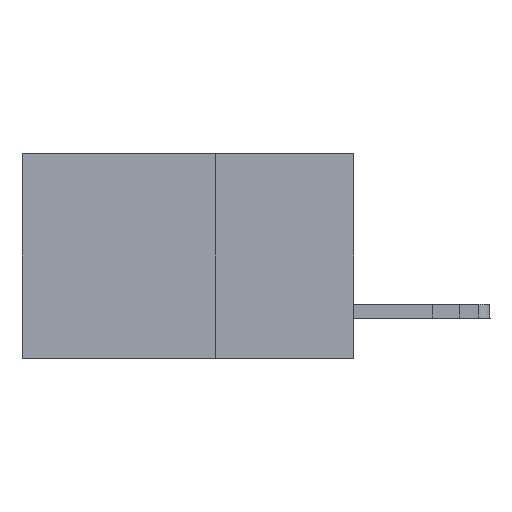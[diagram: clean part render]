
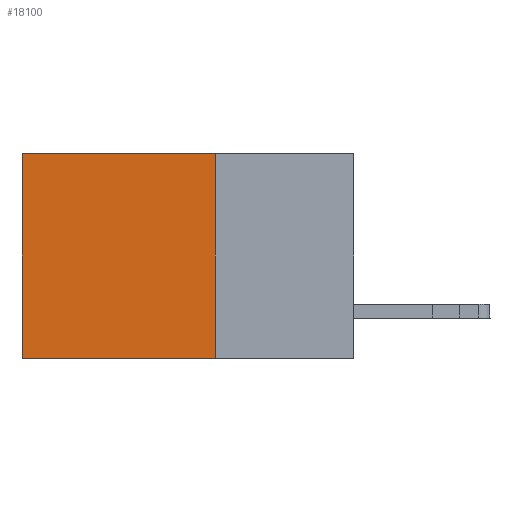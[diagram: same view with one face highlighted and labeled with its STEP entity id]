
A CAD part, left-side view. The second image highlights one B-rep face of the part: STEP entity #18100.
In plain terms, the highlighted planar face has unit normal (-1, 0, 0).
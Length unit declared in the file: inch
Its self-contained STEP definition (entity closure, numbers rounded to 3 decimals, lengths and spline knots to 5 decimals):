
#884 = CARTESIAN_POINT ( 'NONE',  ( 0.2875, 0.25, 0. ) ) ;
#951 = LINE ( 'NONE', #884, #16177 ) ;
#1724 = CARTESIAN_POINT ( 'NONE',  ( 0.2875, 0.6, -0.37 ) ) ;
#5218 = FACE_OUTER_BOUND ( 'NONE', #9682, .T. ) ;
#5630 = VECTOR ( 'NONE', #9436, 39.37008 ) ;
#6949 = VERTEX_POINT ( 'NONE', #14940 ) ;
#7787 = ORIENTED_EDGE ( 'NONE', *, *, #22216, .T. ) ;
#7850 = EDGE_CURVE ( 'NONE', #13435, #17600, #13889, .T. ) ;
#7934 = ORIENTED_EDGE ( 'NONE', *, *, #16994, .F. ) ;
#8490 = CARTESIAN_POINT ( 'NONE',  ( 0.2875, 0.6, 0. ) ) ;
#9195 = ORIENTED_EDGE ( 'NONE', *, *, #7850, .T. ) ;
#9237 = CARTESIAN_POINT ( 'NONE',  ( 0.2875, 0.25, 0. ) ) ;
#9436 = DIRECTION ( 'NONE',  ( 0., 0., -1. ) ) ;
#9438 = CARTESIAN_POINT ( 'NONE',  ( 0.2875, 0.25, -0.37 ) ) ;
#9679 = CARTESIAN_POINT ( 'NONE',  ( 0.2875, 0.6, 0. ) ) ;
#9682 = EDGE_LOOP ( 'NONE', ( #9195, #7934, #17062, #7787 ) ) ;
#9987 = DIRECTION ( 'NONE',  ( 1., 0., 0. ) ) ;
#11471 = LINE ( 'NONE', #23529, #5630 ) ;
#11660 = DIRECTION ( 'NONE',  ( 0., 0., -1. ) ) ;
#12580 = VECTOR ( 'NONE', #21463, 39.37008 ) ;
#13435 = VERTEX_POINT ( 'NONE', #8490 ) ;
#13889 = LINE ( 'NONE', #9679, #24053 ) ;
#14884 = EDGE_CURVE ( 'NONE', #24000, #6949, #11471, .T. ) ;
#14940 = CARTESIAN_POINT ( 'NONE',  ( 0.2875, 0.25, -0.37 ) ) ;
#16177 = VECTOR ( 'NONE', #20763, 39.37008 ) ;
#16994 = EDGE_CURVE ( 'NONE', #6949, #17600, #17285, .T. ) ;
#17062 = ORIENTED_EDGE ( 'NONE', *, *, #14884, .F. ) ;
#17285 = LINE ( 'NONE', #9438, #12580 ) ;
#17600 = VERTEX_POINT ( 'NONE', #1724 ) ;
#18100 = ADVANCED_FACE ( 'NONE', ( #5218 ), #19983, .F. ) ;
#19983 = PLANE ( 'NONE',  #22401 ) ;
#20763 = DIRECTION ( 'NONE',  ( 0., 1., 0. ) ) ;
#21463 = DIRECTION ( 'NONE',  ( 0., 1., 0. ) ) ;
#22025 = CARTESIAN_POINT ( 'NONE',  ( 0.2875, 0.25, 0. ) ) ;
#22216 = EDGE_CURVE ( 'NONE', #24000, #13435, #951, .T. ) ;
#22401 = AXIS2_PLACEMENT_3D ( 'NONE', #22025, #9987, #24088 ) ;
#23529 = CARTESIAN_POINT ( 'NONE',  ( 0.2875, 0.25, 0. ) ) ;
#24000 = VERTEX_POINT ( 'NONE', #9237 ) ;
#24053 = VECTOR ( 'NONE', #11660, 39.37008 ) ;
#24088 = DIRECTION ( 'NONE',  ( 0., 0., -1. ) ) ;
